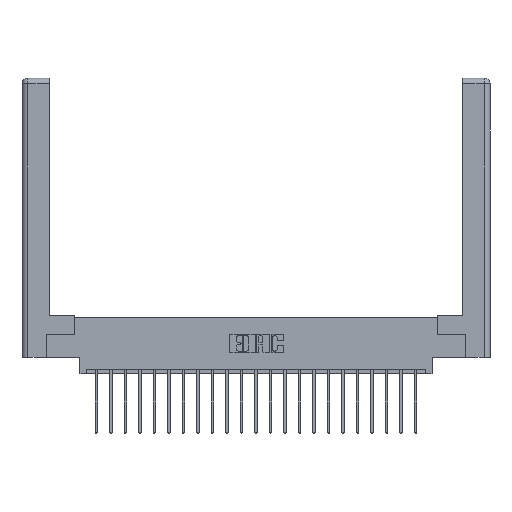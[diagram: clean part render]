
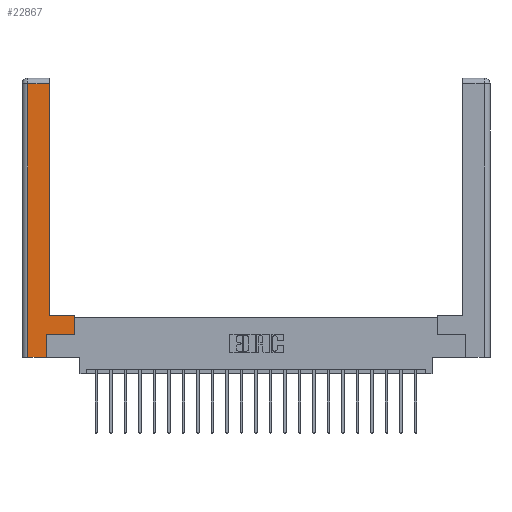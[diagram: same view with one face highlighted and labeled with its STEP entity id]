
A CAD part, top view. The second image highlights one B-rep face of the part: STEP entity #22867.
In plain terms, the highlighted planar face has unit normal (0, 0, 1).
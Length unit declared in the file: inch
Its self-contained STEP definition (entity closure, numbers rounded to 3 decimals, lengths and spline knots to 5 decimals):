
#788 = ORIENTED_EDGE ( 'NONE', *, *, #1344, .T. ) ;
#824 = CARTESIAN_POINT ( 'NONE',  ( 0.0615, 0., 0. ) ) ;
#1069 = FACE_OUTER_BOUND ( 'NONE', #11701, .T. ) ;
#1344 = EDGE_CURVE ( 'NONE', #7950, #11713, #19694, .T. ) ;
#2109 = CARTESIAN_POINT ( 'NONE',  ( 0.265, 0.245, 0. ) ) ;
#2874 = EDGE_CURVE ( 'NONE', #16971, #13634, #5422, .T. ) ;
#3441 = VERTEX_POINT ( 'NONE', #13882 ) ;
#3892 = VECTOR ( 'NONE', #12375, 39.37008 ) ;
#4714 = DIRECTION ( 'NONE',  ( 1., 0., 0. ) ) ;
#4817 = EDGE_CURVE ( 'NONE', #13634, #15960, #14282, .T. ) ;
#4959 = EDGE_CURVE ( 'NONE', #15960, #19012, #8942, .T. ) ;
#5281 = PLANE ( 'NONE',  #13520 ) ;
#5422 = LINE ( 'NONE', #21024, #8487 ) ;
#5788 = CARTESIAN_POINT ( 'NONE',  ( 0.295, 0.45, 0. ) ) ;
#6119 = VECTOR ( 'NONE', #11763, 39.37008 ) ;
#6180 = DIRECTION ( 'NONE',  ( 0., 1., 0. ) ) ;
#7363 = DIRECTION ( 'NONE',  ( -1., 0., 0. ) ) ;
#7740 = VECTOR ( 'NONE', #6180, 39.37008 ) ;
#7950 = VERTEX_POINT ( 'NONE', #10068 ) ;
#8487 = VECTOR ( 'NONE', #15751, 39.37008 ) ;
#8563 = ORIENTED_EDGE ( 'NONE', *, *, #9746, .T. ) ;
#8814 = VECTOR ( 'NONE', #14094, 39.37008 ) ;
#8927 = EDGE_CURVE ( 'NONE', #19012, #7950, #17007, .T. ) ;
#8942 = LINE ( 'NONE', #22584, #13151 ) ;
#9746 = EDGE_CURVE ( 'NONE', #11713, #3441, #17802, .T. ) ;
#9753 = CARTESIAN_POINT ( 'NONE',  ( 0.295, 2.94, 0. ) ) ;
#10068 = CARTESIAN_POINT ( 'NONE',  ( 0.265, 0.245, 0. ) ) ;
#10401 = EDGE_CURVE ( 'NONE', #3441, #20791, #14730, .T. ) ;
#11701 = EDGE_LOOP ( 'NONE', ( #17213, #20176, #21920, #12554, #22124, #788, #8563, #16397 ) ) ;
#11713 = VERTEX_POINT ( 'NONE', #19309 ) ;
#11763 = DIRECTION ( 'NONE',  ( 0., 1., 0. ) ) ;
#12375 = DIRECTION ( 'NONE',  ( 0., -1., 0. ) ) ;
#12481 = DIRECTION ( 'NONE',  ( 0., 0., -1. ) ) ;
#12554 = ORIENTED_EDGE ( 'NONE', *, *, #4959, .T. ) ;
#12771 = DIRECTION ( 'NONE',  ( 0., 1., 0. ) ) ;
#12997 = DIRECTION ( 'NONE',  ( -1., 0., 0. ) ) ;
#13151 = VECTOR ( 'NONE', #4714, 39.37008 ) ;
#13429 = LINE ( 'NONE', #20632, #6119 ) ;
#13520 = AXIS2_PLACEMENT_3D ( 'NONE', #19561, #12481, #7363 ) ;
#13610 = VECTOR ( 'NONE', #12997, 39.37008 ) ;
#13634 = VERTEX_POINT ( 'NONE', #20273 ) ;
#13882 = CARTESIAN_POINT ( 'NONE',  ( 0.565, 0.45, 0. ) ) ;
#14094 = DIRECTION ( 'NONE',  ( 1., 0., 0. ) ) ;
#14282 = LINE ( 'NONE', #14946, #3892 ) ;
#14730 = LINE ( 'NONE', #5788, #13610 ) ;
#14946 = CARTESIAN_POINT ( 'NONE',  ( 0.0615, 0., 0. ) ) ;
#15751 = DIRECTION ( 'NONE',  ( -1., 0., 0. ) ) ;
#15960 = VERTEX_POINT ( 'NONE', #824 ) ;
#16147 = CARTESIAN_POINT ( 'NONE',  ( 0.295, 0.45, 0. ) ) ;
#16397 = ORIENTED_EDGE ( 'NONE', *, *, #10401, .T. ) ;
#16971 = VERTEX_POINT ( 'NONE', #9753 ) ;
#17007 = LINE ( 'NONE', #2109, #17823 ) ;
#17123 = CARTESIAN_POINT ( 'NONE',  ( 0.265, 0., 0. ) ) ;
#17213 = ORIENTED_EDGE ( 'NONE', *, *, #17223, .T. ) ;
#17223 = EDGE_CURVE ( 'NONE', #20791, #16971, #13429, .T. ) ;
#17802 = LINE ( 'NONE', #21890, #7740 ) ;
#17823 = VECTOR ( 'NONE', #12771, 39.37008 ) ;
#19012 = VERTEX_POINT ( 'NONE', #17123 ) ;
#19309 = CARTESIAN_POINT ( 'NONE',  ( 0.565, 0.245, 0. ) ) ;
#19526 = CARTESIAN_POINT ( 'NONE',  ( 0.565, 0.245, 0. ) ) ;
#19561 = CARTESIAN_POINT ( 'NONE',  ( 0., 0., 0. ) ) ;
#19694 = LINE ( 'NONE', #19526, #8814 ) ;
#20176 = ORIENTED_EDGE ( 'NONE', *, *, #2874, .T. ) ;
#20273 = CARTESIAN_POINT ( 'NONE',  ( 0.0615, 2.94, 0. ) ) ;
#20632 = CARTESIAN_POINT ( 'NONE',  ( 0.295, 3., 0. ) ) ;
#20791 = VERTEX_POINT ( 'NONE', #16147 ) ;
#21024 = CARTESIAN_POINT ( 'NONE',  ( 0.0615, 2.94, 0. ) ) ;
#21890 = CARTESIAN_POINT ( 'NONE',  ( 0.565, 0.45, 0. ) ) ;
#21920 = ORIENTED_EDGE ( 'NONE', *, *, #4817, .T. ) ;
#22124 = ORIENTED_EDGE ( 'NONE', *, *, #8927, .T. ) ;
#22584 = CARTESIAN_POINT ( 'NONE',  ( 0.265, 0., 0. ) ) ;
#22867 = ADVANCED_FACE ( 'NONE', ( #1069 ), #5281, .F. ) ;
